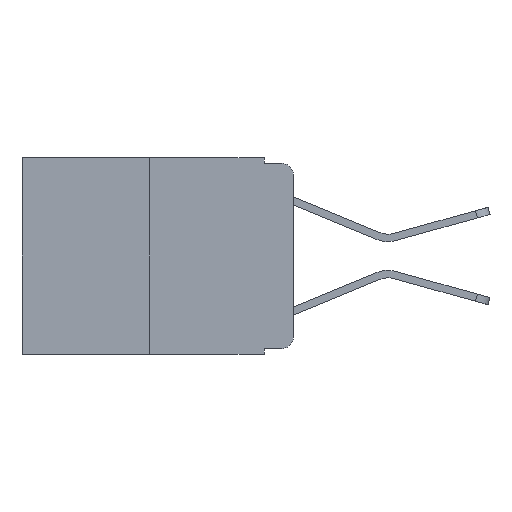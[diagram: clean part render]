
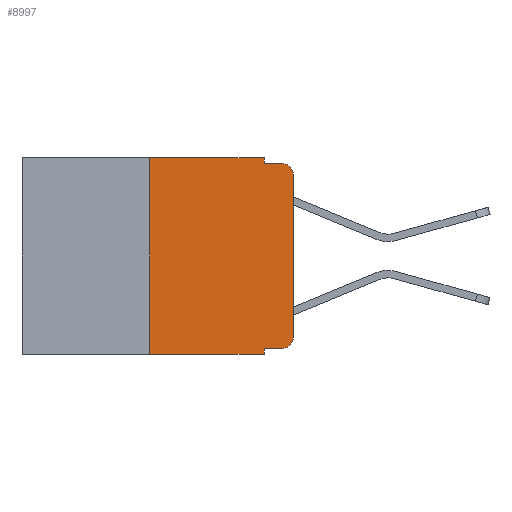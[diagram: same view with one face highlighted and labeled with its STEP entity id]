
A CAD part, left-side view. The second image highlights one B-rep face of the part: STEP entity #8997.
In plain terms, the highlighted planar face has unit normal (-1, 0, 0).
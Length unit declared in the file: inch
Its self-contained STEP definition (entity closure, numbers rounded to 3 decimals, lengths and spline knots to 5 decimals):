
#207 = AXIS2_PLACEMENT_3D ( 'NONE', #12932, #10569, #9676 ) ;
#275 = LINE ( 'NONE', #13048, #12865 ) ;
#359 = VERTEX_POINT ( 'NONE', #10607 ) ;
#731 = CARTESIAN_POINT ( 'NONE',  ( 0., 0.051, 0. ) ) ;
#781 = CARTESIAN_POINT ( 'NONE',  ( 0., 0.02, -0.01 ) ) ;
#1056 = VECTOR ( 'NONE', #6394, 39.37008 ) ;
#1345 = EDGE_CURVE ( 'NONE', #9140, #13222, #275, .T. ) ;
#1372 = CARTESIAN_POINT ( 'NONE',  ( 0., 0.02, -0.03 ) ) ;
#1374 = ORIENTED_EDGE ( 'NONE', *, *, #8380, .F. ) ;
#1535 = VECTOR ( 'NONE', #10068, 39.37008 ) ;
#2571 = DIRECTION ( 'NONE',  ( 0., -1., 0. ) ) ;
#2802 = CARTESIAN_POINT ( 'NONE',  ( 0., 0.051, -0.01 ) ) ;
#2834 = EDGE_CURVE ( 'NONE', #3883, #10597, #7837, .T. ) ;
#3061 = AXIS2_PLACEMENT_3D ( 'NONE', #11580, #10677, #3246 ) ;
#3178 = LINE ( 'NONE', #5198, #6664 ) ;
#3208 = PLANE ( 'NONE',  #207 ) ;
#3246 = DIRECTION ( 'NONE',  ( 0., 0., -1. ) ) ;
#3274 = CARTESIAN_POINT ( 'NONE',  ( 0., 0.051, -0.343 ) ) ;
#3517 = VERTEX_POINT ( 'NONE', #5171 ) ;
#3716 = DIRECTION ( 'NONE',  ( 0., 0., -1. ) ) ;
#3866 = ORIENTED_EDGE ( 'NONE', *, *, #9764, .T. ) ;
#3875 = ORIENTED_EDGE ( 'NONE', *, *, #6988, .F. ) ;
#3883 = VERTEX_POINT ( 'NONE', #7076 ) ;
#3892 = EDGE_CURVE ( 'NONE', #13314, #13222, #12568, .T. ) ;
#3969 = ORIENTED_EDGE ( 'NONE', *, *, #8109, .T. ) ;
#3994 = ORIENTED_EDGE ( 'NONE', *, *, #1345, .T. ) ;
#4074 = VECTOR ( 'NONE', #2571, 39.37008 ) ;
#4246 = CARTESIAN_POINT ( 'NONE',  ( 0., 0.051, 0. ) ) ;
#5113 = CARTESIAN_POINT ( 'NONE',  ( 0., 0.051, -0.333 ) ) ;
#5154 = VERTEX_POINT ( 'NONE', #781 ) ;
#5171 = CARTESIAN_POINT ( 'NONE',  ( 0., 0.051, -0.01 ) ) ;
#5198 = CARTESIAN_POINT ( 'NONE',  ( 0., 0.25, 0. ) ) ;
#5639 = CARTESIAN_POINT ( 'NONE',  ( 0., 0.051, -0.333 ) ) ;
#5738 = VERTEX_POINT ( 'NONE', #6027 ) ;
#5753 = CARTESIAN_POINT ( 'NONE',  ( 0., 0.473, 0. ) ) ;
#5826 = ORIENTED_EDGE ( 'NONE', *, *, #12181, .F. ) ;
#5971 = DIRECTION ( 'NONE',  ( 0., 0., -1. ) ) ;
#6027 = CARTESIAN_POINT ( 'NONE',  ( 0., 0.02, -0.333 ) ) ;
#6367 = VECTOR ( 'NONE', #10309, 39.37008 ) ;
#6394 = DIRECTION ( 'NONE',  ( 0., 0., 1. ) ) ;
#6519 = DIRECTION ( 'NONE',  ( 0., -1., 0. ) ) ;
#6664 = VECTOR ( 'NONE', #7336, 39.37008 ) ;
#6904 = LINE ( 'NONE', #731, #1535 ) ;
#6988 = EDGE_CURVE ( 'NONE', #3517, #5154, #10512, .T. ) ;
#7076 = CARTESIAN_POINT ( 'NONE',  ( 0., 0.25, 0. ) ) ;
#7110 = EDGE_CURVE ( 'NONE', #359, #10994, #12654, .T. ) ;
#7250 = ORIENTED_EDGE ( 'NONE', *, *, #9630, .T. ) ;
#7251 = CARTESIAN_POINT ( 'NONE',  ( 0., 0., -0.03 ) ) ;
#7289 = CARTESIAN_POINT ( 'NONE',  ( 0., 0.051, 0. ) ) ;
#7336 = DIRECTION ( 'NONE',  ( 0., 0., 1. ) ) ;
#7374 = CARTESIAN_POINT ( 'NONE',  ( 0., 0., 0. ) ) ;
#7570 = FACE_OUTER_BOUND ( 'NONE', #10351, .T. ) ;
#7722 = CIRCLE ( 'NONE', #3061, 0.02 ) ;
#7766 = ORIENTED_EDGE ( 'NONE', *, *, #2834, .F. ) ;
#7837 = LINE ( 'NONE', #5753, #4074 ) ;
#7917 = ORIENTED_EDGE ( 'NONE', *, *, #3892, .F. ) ;
#7940 = LINE ( 'NONE', #5113, #13317 ) ;
#8109 = EDGE_CURVE ( 'NONE', #5738, #359, #7722, .T. ) ;
#8380 = EDGE_CURVE ( 'NONE', #10597, #3517, #6904, .T. ) ;
#8997 = ADVANCED_FACE ( 'NONE', ( #7570 ), #3208, .F. ) ;
#9006 = DIRECTION ( 'NONE',  ( -1., 0., 0. ) ) ;
#9140 = VERTEX_POINT ( 'NONE', #10900 ) ;
#9551 = CIRCLE ( 'NONE', #9997, 0.02 ) ;
#9630 = EDGE_CURVE ( 'NONE', #10994, #5154, #9551, .T. ) ;
#9676 = DIRECTION ( 'NONE',  ( 0., 0., -1. ) ) ;
#9764 = EDGE_CURVE ( 'NONE', #13314, #5738, #7940, .T. ) ;
#9997 = AXIS2_PLACEMENT_3D ( 'NONE', #1372, #9006, #3716 ) ;
#10068 = DIRECTION ( 'NONE',  ( 0., 0., -1. ) ) ;
#10309 = DIRECTION ( 'NONE',  ( 0., -1., 0. ) ) ;
#10351 = EDGE_LOOP ( 'NONE', ( #12698, #7250, #3875, #1374, #7766, #5826, #3994, #7917, #3866, #3969 ) ) ;
#10512 = LINE ( 'NONE', #2802, #6367 ) ;
#10569 = DIRECTION ( 'NONE',  ( 1., 0., 0. ) ) ;
#10597 = VERTEX_POINT ( 'NONE', #4246 ) ;
#10607 = CARTESIAN_POINT ( 'NONE',  ( 0., 0., -0.313 ) ) ;
#10677 = DIRECTION ( 'NONE',  ( -1., 0., 0. ) ) ;
#10900 = CARTESIAN_POINT ( 'NONE',  ( 0., 0.25, -0.343 ) ) ;
#10994 = VERTEX_POINT ( 'NONE', #7251 ) ;
#11267 = VECTOR ( 'NONE', #5971, 39.37008 ) ;
#11580 = CARTESIAN_POINT ( 'NONE',  ( 0., 0.02, -0.313 ) ) ;
#12181 = EDGE_CURVE ( 'NONE', #9140, #3883, #3178, .T. ) ;
#12568 = LINE ( 'NONE', #7289, #11267 ) ;
#12654 = LINE ( 'NONE', #7374, #1056 ) ;
#12698 = ORIENTED_EDGE ( 'NONE', *, *, #7110, .T. ) ;
#12865 = VECTOR ( 'NONE', #6519, 39.37008 ) ;
#12932 = CARTESIAN_POINT ( 'NONE',  ( 0., 0.473, 0. ) ) ;
#13048 = CARTESIAN_POINT ( 'NONE',  ( 0., 0.473, -0.343 ) ) ;
#13222 = VERTEX_POINT ( 'NONE', #3274 ) ;
#13314 = VERTEX_POINT ( 'NONE', #5639 ) ;
#13317 = VECTOR ( 'NONE', #13598, 39.37008 ) ;
#13598 = DIRECTION ( 'NONE',  ( 0., -1., 0. ) ) ;
